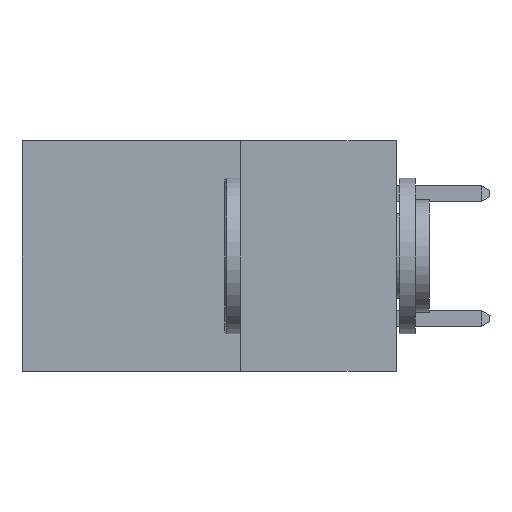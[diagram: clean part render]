
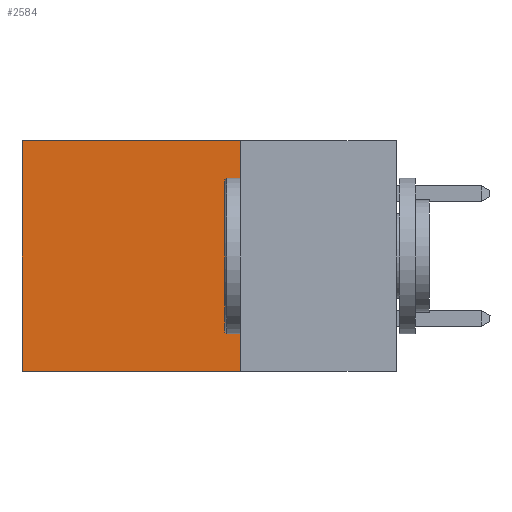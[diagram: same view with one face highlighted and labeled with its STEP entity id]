
A CAD part, left-side view. The second image highlights one B-rep face of the part: STEP entity #2584.
In plain terms, the highlighted planar face has unit normal (-1, 0, 0).
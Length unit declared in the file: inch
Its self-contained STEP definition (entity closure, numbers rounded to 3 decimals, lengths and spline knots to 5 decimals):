
#18 = DIRECTION ( 'NONE',  ( 0., 1., 0. ) ) ;
#37 = CARTESIAN_POINT ( 'NONE',  ( 0.2615, 0.6, -0.37 ) ) ;
#334 = LINE ( 'NONE', #7268, #10088 ) ;
#832 = CARTESIAN_POINT ( 'NONE',  ( 0.2615, 0.25, 0. ) ) ;
#1029 = CARTESIAN_POINT ( 'NONE',  ( 0.2615, 0.6, 0. ) ) ;
#1680 = CARTESIAN_POINT ( 'NONE',  ( 0.2615, 0.25, 0. ) ) ;
#1913 = CARTESIAN_POINT ( 'NONE',  ( 0.2615, 0.25, -0.37 ) ) ;
#2492 = CARTESIAN_POINT ( 'NONE',  ( 0.2615, 0.6, -0.37 ) ) ;
#2493 = DIRECTION ( 'NONE',  ( 0., 1., 0. ) ) ;
#2584 = ADVANCED_FACE ( 'NONE', ( #4572 ), #2742, .F. ) ;
#2742 = PLANE ( 'NONE',  #7442 ) ;
#3096 = ORIENTED_EDGE ( 'NONE', *, *, #6731, .T. ) ;
#3604 = ORIENTED_EDGE ( 'NONE', *, *, #9256, .F. ) ;
#4036 = LINE ( 'NONE', #1680, #9995 ) ;
#4059 = EDGE_CURVE ( 'NONE', #9265, #7386, #6457, .T. ) ;
#4298 = VECTOR ( 'NONE', #4862, 39.37008 ) ;
#4572 = FACE_OUTER_BOUND ( 'NONE', #9824, .T. ) ;
#4755 = ORIENTED_EDGE ( 'NONE', *, *, #4059, .F. ) ;
#4813 = VERTEX_POINT ( 'NONE', #37 ) ;
#4862 = DIRECTION ( 'NONE',  ( 0., 0., -1. ) ) ;
#5125 = ORIENTED_EDGE ( 'NONE', *, *, #8201, .T. ) ;
#5853 = VECTOR ( 'NONE', #6562, 39.37008 ) ;
#6010 = DIRECTION ( 'NONE',  ( 1., 0., 0. ) ) ;
#6099 = LINE ( 'NONE', #2492, #5853 ) ;
#6457 = LINE ( 'NONE', #1913, #4298 ) ;
#6517 = CARTESIAN_POINT ( 'NONE',  ( 0.2615, 0.25, -0.37 ) ) ;
#6562 = DIRECTION ( 'NONE',  ( 0., 0., -1. ) ) ;
#6731 = EDGE_CURVE ( 'NONE', #6879, #4813, #6099, .T. ) ;
#6879 = VERTEX_POINT ( 'NONE', #1029 ) ;
#7268 = CARTESIAN_POINT ( 'NONE',  ( 0.2615, 0.25, -0.37 ) ) ;
#7386 = VERTEX_POINT ( 'NONE', #6517 ) ;
#7418 = DIRECTION ( 'NONE',  ( 0., 0., -1. ) ) ;
#7442 = AXIS2_PLACEMENT_3D ( 'NONE', #8006, #6010, #7418 ) ;
#8006 = CARTESIAN_POINT ( 'NONE',  ( 0.2615, 0.25, -0.37 ) ) ;
#8201 = EDGE_CURVE ( 'NONE', #9265, #6879, #4036, .T. ) ;
#9256 = EDGE_CURVE ( 'NONE', #7386, #4813, #334, .T. ) ;
#9265 = VERTEX_POINT ( 'NONE', #832 ) ;
#9824 = EDGE_LOOP ( 'NONE', ( #3096, #3604, #4755, #5125 ) ) ;
#9995 = VECTOR ( 'NONE', #2493, 39.37008 ) ;
#10088 = VECTOR ( 'NONE', #18, 39.37008 ) ;
